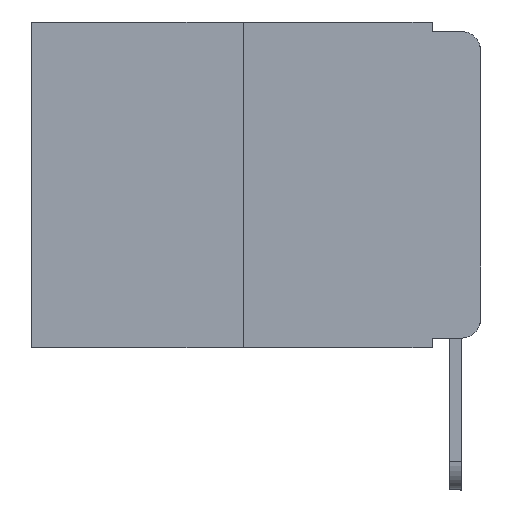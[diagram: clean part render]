
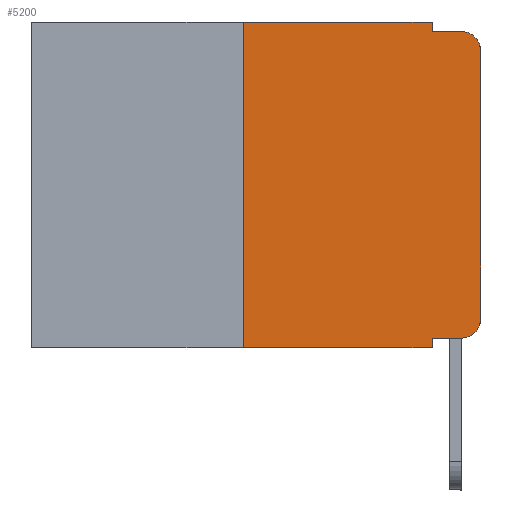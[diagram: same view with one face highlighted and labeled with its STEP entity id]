
A CAD part, left-side view. The second image highlights one B-rep face of the part: STEP entity #5200.
In plain terms, the highlighted planar face has unit normal (-1, 0, 0).
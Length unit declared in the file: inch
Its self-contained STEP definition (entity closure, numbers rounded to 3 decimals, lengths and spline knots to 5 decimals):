
#702 = VERTEX_POINT ( 'NONE', #8317 ) ;
#1154 = ORIENTED_EDGE ( 'NONE', *, *, #12553, .F. ) ;
#1265 = DIRECTION ( 'NONE',  ( 0., 0., 1. ) ) ;
#1466 = ORIENTED_EDGE ( 'NONE', *, *, #15681, .F. ) ;
#1600 = VERTEX_POINT ( 'NONE', #2602 ) ;
#1808 = CARTESIAN_POINT ( 'NONE',  ( 0., 0.25, 0. ) ) ;
#1974 = LINE ( 'NONE', #14970, #15593 ) ;
#2044 = CIRCLE ( 'NONE', #10957, 0.02 ) ;
#2199 = PLANE ( 'NONE',  #6605 ) ;
#2203 = CARTESIAN_POINT ( 'NONE',  ( 0., 0., -0.03 ) ) ;
#2235 = CARTESIAN_POINT ( 'NONE',  ( 0., 0.051, -0.333 ) ) ;
#2449 = CARTESIAN_POINT ( 'NONE',  ( 0., 0.25, 0. ) ) ;
#2602 = CARTESIAN_POINT ( 'NONE',  ( 0., 0.051, -0.01 ) ) ;
#2751 = CIRCLE ( 'NONE', #4842, 0.02 ) ;
#3604 = VECTOR ( 'NONE', #15573, 39.37008 ) ;
#3693 = EDGE_CURVE ( 'NONE', #4067, #6466, #18153, .T. ) ;
#3844 = LINE ( 'NONE', #8126, #11358 ) ;
#3914 = CARTESIAN_POINT ( 'NONE',  ( 0., 0.02, -0.03 ) ) ;
#3959 = LINE ( 'NONE', #10937, #7195 ) ;
#3982 = EDGE_LOOP ( 'NONE', ( #17965, #11724, #1154, #7067, #6120, #1466, #8619, #14946, #5598, #15317 ) ) ;
#4067 = VERTEX_POINT ( 'NONE', #5881 ) ;
#4483 = EDGE_CURVE ( 'NONE', #6466, #702, #2044, .T. ) ;
#4649 = DIRECTION ( 'NONE',  ( 0., -1., 0. ) ) ;
#4742 = CARTESIAN_POINT ( 'NONE',  ( 0., 0.02, -0.313 ) ) ;
#4842 = AXIS2_PLACEMENT_3D ( 'NONE', #4742, #7629, #6522 ) ;
#5200 = ADVANCED_FACE ( 'NONE', ( #17518 ), #2199, .F. ) ;
#5259 = CARTESIAN_POINT ( 'NONE',  ( 0., 0.051, -0.343 ) ) ;
#5598 = ORIENTED_EDGE ( 'NONE', *, *, #12317, .T. ) ;
#5660 = DIRECTION ( 'NONE',  ( 0., 0., -1. ) ) ;
#5881 = CARTESIAN_POINT ( 'NONE',  ( 0., 0., -0.313 ) ) ;
#6087 = VECTOR ( 'NONE', #5660, 39.37008 ) ;
#6120 = ORIENTED_EDGE ( 'NONE', *, *, #9807, .F. ) ;
#6466 = VERTEX_POINT ( 'NONE', #2203 ) ;
#6522 = DIRECTION ( 'NONE',  ( 0., 0., -1. ) ) ;
#6605 = AXIS2_PLACEMENT_3D ( 'NONE', #14730, #13249, #9178 ) ;
#6803 = DIRECTION ( 'NONE',  ( -1., 0., 0. ) ) ;
#6961 = LINE ( 'NONE', #11413, #3604 ) ;
#7067 = ORIENTED_EDGE ( 'NONE', *, *, #13255, .F. ) ;
#7133 = LINE ( 'NONE', #15462, #6087 ) ;
#7195 = VECTOR ( 'NONE', #16574, 39.37008 ) ;
#7305 = VERTEX_POINT ( 'NONE', #15987 ) ;
#7569 = VECTOR ( 'NONE', #13138, 39.37008 ) ;
#7629 = DIRECTION ( 'NONE',  ( -1., 0., 0. ) ) ;
#7678 = LINE ( 'NONE', #1808, #7569 ) ;
#7752 = DIRECTION ( 'NONE',  ( 0., -1., 0. ) ) ;
#8126 = CARTESIAN_POINT ( 'NONE',  ( 0., 0.051, 0. ) ) ;
#8242 = VERTEX_POINT ( 'NONE', #5259 ) ;
#8317 = CARTESIAN_POINT ( 'NONE',  ( 0., 0.02, -0.01 ) ) ;
#8403 = VERTEX_POINT ( 'NONE', #15910 ) ;
#8466 = DIRECTION ( 'NONE',  ( 0., 0., -1. ) ) ;
#8619 = ORIENTED_EDGE ( 'NONE', *, *, #18200, .T. ) ;
#9178 = DIRECTION ( 'NONE',  ( 0., 0., -1. ) ) ;
#9750 = CARTESIAN_POINT ( 'NONE',  ( 0., 0.25, -0.343 ) ) ;
#9807 = EDGE_CURVE ( 'NONE', #11600, #8403, #3959, .T. ) ;
#10588 = LINE ( 'NONE', #17445, #13683 ) ;
#10937 = CARTESIAN_POINT ( 'NONE',  ( 0., 0.473, 0. ) ) ;
#10941 = CARTESIAN_POINT ( 'NONE',  ( 0., 0., 0. ) ) ;
#10957 = AXIS2_PLACEMENT_3D ( 'NONE', #3914, #6803, #8466 ) ;
#11358 = VECTOR ( 'NONE', #12295, 39.37008 ) ;
#11413 = CARTESIAN_POINT ( 'NONE',  ( 0., 0.051, -0.01 ) ) ;
#11600 = VERTEX_POINT ( 'NONE', #2449 ) ;
#11724 = ORIENTED_EDGE ( 'NONE', *, *, #4483, .T. ) ;
#12295 = DIRECTION ( 'NONE',  ( 0., 0., -1. ) ) ;
#12317 = EDGE_CURVE ( 'NONE', #16837, #7305, #10588, .T. ) ;
#12553 = EDGE_CURVE ( 'NONE', #1600, #702, #6961, .T. ) ;
#12633 = VERTEX_POINT ( 'NONE', #9750 ) ;
#13138 = DIRECTION ( 'NONE',  ( 0., 0., 1. ) ) ;
#13249 = DIRECTION ( 'NONE',  ( 1., 0., 0. ) ) ;
#13255 = EDGE_CURVE ( 'NONE', #8403, #1600, #3844, .T. ) ;
#13584 = EDGE_CURVE ( 'NONE', #7305, #4067, #2751, .T. ) ;
#13683 = VECTOR ( 'NONE', #4649, 39.37008 ) ;
#14730 = CARTESIAN_POINT ( 'NONE',  ( 0., 0.473, 0. ) ) ;
#14946 = ORIENTED_EDGE ( 'NONE', *, *, #15585, .F. ) ;
#14970 = CARTESIAN_POINT ( 'NONE',  ( 0., 0.473, -0.343 ) ) ;
#15317 = ORIENTED_EDGE ( 'NONE', *, *, #13584, .T. ) ;
#15462 = CARTESIAN_POINT ( 'NONE',  ( 0., 0.051, 0. ) ) ;
#15573 = DIRECTION ( 'NONE',  ( 0., -1., 0. ) ) ;
#15585 = EDGE_CURVE ( 'NONE', #16837, #8242, #7133, .T. ) ;
#15593 = VECTOR ( 'NONE', #7752, 39.37008 ) ;
#15681 = EDGE_CURVE ( 'NONE', #12633, #11600, #7678, .T. ) ;
#15910 = CARTESIAN_POINT ( 'NONE',  ( 0., 0.051, 0. ) ) ;
#15987 = CARTESIAN_POINT ( 'NONE',  ( 0., 0.02, -0.333 ) ) ;
#16574 = DIRECTION ( 'NONE',  ( 0., -1., 0. ) ) ;
#16837 = VERTEX_POINT ( 'NONE', #2235 ) ;
#17138 = VECTOR ( 'NONE', #1265, 39.37008 ) ;
#17445 = CARTESIAN_POINT ( 'NONE',  ( 0., 0.051, -0.333 ) ) ;
#17518 = FACE_OUTER_BOUND ( 'NONE', #3982, .T. ) ;
#17965 = ORIENTED_EDGE ( 'NONE', *, *, #3693, .T. ) ;
#18153 = LINE ( 'NONE', #10941, #17138 ) ;
#18200 = EDGE_CURVE ( 'NONE', #12633, #8242, #1974, .T. ) ;
